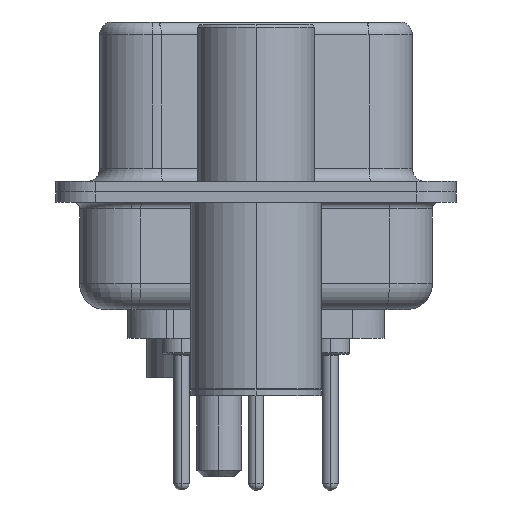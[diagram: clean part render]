
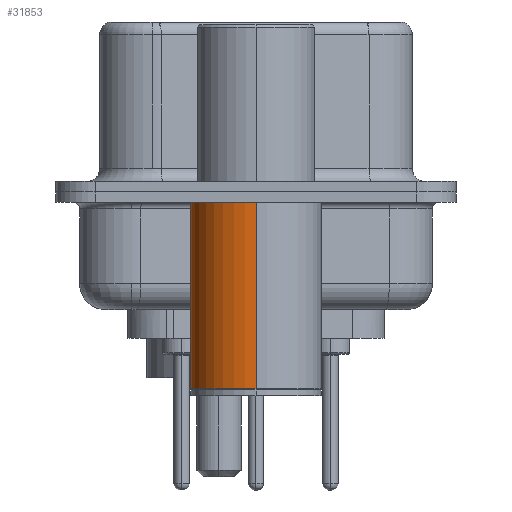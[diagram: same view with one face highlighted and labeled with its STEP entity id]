
A CAD part, left-side view. The second image highlights one B-rep face of the part: STEP entity #31853.
In plain terms, the highlighted cylindrical face has radius 2.5 mm (diameter 5 mm), a partial arc.
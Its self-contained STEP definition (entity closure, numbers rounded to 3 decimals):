
#1199 = DIRECTION ( 'NONE',  ( 1., 0., 0. ) ) ;
#1608 = CARTESIAN_POINT ( 'NONE',  ( 0., 0., 0.581 ) ) ;
#2223 = DIRECTION ( 'NONE',  ( 0., 0., 1. ) ) ;
#2404 = AXIS2_PLACEMENT_3D ( 'NONE', #34977, #17942, #1199 ) ;
#3036 = EDGE_CURVE ( 'NONE', #29875, #23341, #28646, .T. ) ;
#3505 = CARTESIAN_POINT ( 'NONE',  ( 0., 0., -7.525 ) ) ;
#4344 = LINE ( 'NONE', #18936, #33436 ) ;
#4438 = DIRECTION ( 'NONE',  ( 1., 0., 0. ) ) ;
#5247 = CARTESIAN_POINT ( 'NONE',  ( -2.5, 0., -7.525 ) ) ;
#5675 = CARTESIAN_POINT ( 'NONE',  ( 2.5, 0., -7.525 ) ) ;
#5880 = CARTESIAN_POINT ( 'NONE',  ( -2.5, 0., 0.581 ) ) ;
#6271 = VECTOR ( 'NONE', #32675, 1000. ) ;
#6345 = DIRECTION ( 'NONE',  ( 1., 0., 0. ) ) ;
#7027 = CYLINDRICAL_SURFACE ( 'NONE', #9902, 2.5 ) ;
#7907 = FACE_OUTER_BOUND ( 'NONE', #34755, .T. ) ;
#7985 = VERTEX_POINT ( 'NONE', #5675 ) ;
#9902 = AXIS2_PLACEMENT_3D ( 'NONE', #1608, #21121, #4438 ) ;
#10350 = CARTESIAN_POINT ( 'NONE',  ( 2.5, 0., -0.4 ) ) ;
#11271 = VERTEX_POINT ( 'NONE', #10350 ) ;
#16875 = CIRCLE ( 'NONE', #2404, 2.5 ) ;
#17668 = ORIENTED_EDGE ( 'NONE', *, *, #28203, .T. ) ;
#17942 = DIRECTION ( 'NONE',  ( 0., 0., 1. ) ) ;
#18936 = CARTESIAN_POINT ( 'NONE',  ( 2.5, 0., 0.581 ) ) ;
#21121 = DIRECTION ( 'NONE',  ( 0., 0., 1. ) ) ;
#22469 = CARTESIAN_POINT ( 'NONE',  ( -2.5, 0., -0.4 ) ) ;
#22776 = ORIENTED_EDGE ( 'NONE', *, *, #3036, .T. ) ;
#23036 = DIRECTION ( 'NONE',  ( 0., 0., 1. ) ) ;
#23341 = VERTEX_POINT ( 'NONE', #22469 ) ;
#25553 = ORIENTED_EDGE ( 'NONE', *, *, #32014, .F. ) ;
#27199 = AXIS2_PLACEMENT_3D ( 'NONE', #3505, #23036, #6345 ) ;
#28203 = EDGE_CURVE ( 'NONE', #7985, #29875, #28907, .T. ) ;
#28541 = ORIENTED_EDGE ( 'NONE', *, *, #33961, .F. ) ;
#28646 = LINE ( 'NONE', #5880, #6271 ) ;
#28907 = CIRCLE ( 'NONE', #27199, 2.5 ) ;
#29875 = VERTEX_POINT ( 'NONE', #5247 ) ;
#31853 = ADVANCED_FACE ( 'NONE', ( #7907 ), #7027, .T. ) ;
#32014 = EDGE_CURVE ( 'NONE', #7985, #11271, #4344, .T. ) ;
#32675 = DIRECTION ( 'NONE',  ( 0., 0., 1. ) ) ;
#33436 = VECTOR ( 'NONE', #2223, 1000. ) ;
#33961 = EDGE_CURVE ( 'NONE', #11271, #23341, #16875, .T. ) ;
#34755 = EDGE_LOOP ( 'NONE', ( #17668, #22776, #28541, #25553 ) ) ;
#34977 = CARTESIAN_POINT ( 'NONE',  ( 0., 0., -0.4 ) ) ;
